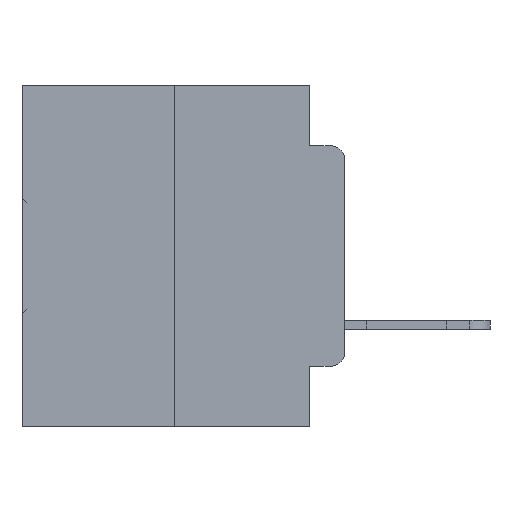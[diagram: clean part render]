
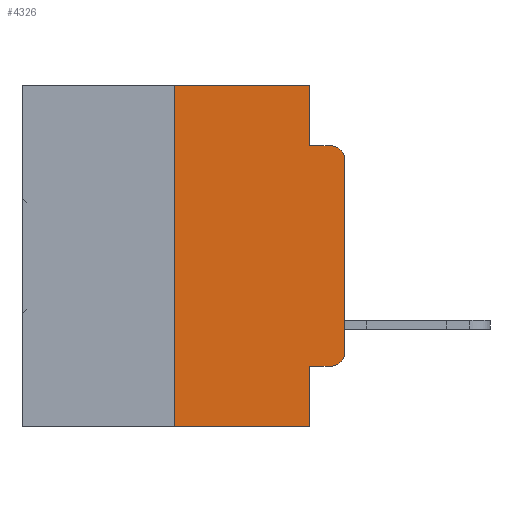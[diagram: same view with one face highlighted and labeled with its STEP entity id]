
A CAD part, left-side view. The second image highlights one B-rep face of the part: STEP entity #4326.
In plain terms, the highlighted planar face has unit normal (-1, 0, 0).
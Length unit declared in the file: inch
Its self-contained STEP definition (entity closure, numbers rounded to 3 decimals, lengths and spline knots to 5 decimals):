
#332 = AXIS2_PLACEMENT_3D ( 'NONE', #28233, #28137, #28130 ) ;
#781 = VECTOR ( 'NONE', #5987, 39.37008 ) ;
#976 = DIRECTION ( 'NONE',  ( 0., -1., 0. ) ) ;
#1057 = CARTESIAN_POINT ( 'NONE',  ( 0., 0.25, -0.5 ) ) ;
#1423 = ORIENTED_EDGE ( 'NONE', *, *, #20901, .F. ) ;
#1630 = CARTESIAN_POINT ( 'NONE',  ( 0., 0., -0.1085 ) ) ;
#2829 = ORIENTED_EDGE ( 'NONE', *, *, #20989, .F. ) ;
#3042 = ORIENTED_EDGE ( 'NONE', *, *, #15015, .F. ) ;
#3251 = EDGE_LOOP ( 'NONE', ( #8736, #9298, #1423, #2829, #3042, #3674, #5039, #5368, #6458, #7933 ) ) ;
#3662 = CARTESIAN_POINT ( 'NONE',  ( 0., 0.051, -0.0885 ) ) ;
#3674 = ORIENTED_EDGE ( 'NONE', *, *, #21372, .F. ) ;
#4326 = ADVANCED_FACE ( 'NONE', ( #28482 ), #28453, .F. ) ;
#5039 = ORIENTED_EDGE ( 'NONE', *, *, #16620, .T. ) ;
#5217 = CARTESIAN_POINT ( 'NONE',  ( 0., 0.473, -0.5 ) ) ;
#5368 = ORIENTED_EDGE ( 'NONE', *, *, #21465, .F. ) ;
#5386 = VECTOR ( 'NONE', #23985, 39.37008 ) ;
#5987 = DIRECTION ( 'NONE',  ( 0., 0., 1. ) ) ;
#6069 = CARTESIAN_POINT ( 'NONE',  ( 0., 0., 0. ) ) ;
#6242 = VECTOR ( 'NONE', #976, 39.37008 ) ;
#6410 = LINE ( 'NONE', #18366, #19585 ) ;
#6458 = ORIENTED_EDGE ( 'NONE', *, *, #21473, .T. ) ;
#7432 = VERTEX_POINT ( 'NONE', #24612 ) ;
#7849 = VERTEX_POINT ( 'NONE', #14392 ) ;
#7933 = ORIENTED_EDGE ( 'NONE', *, *, #21521, .T. ) ;
#8736 = ORIENTED_EDGE ( 'NONE', *, *, #19960, .T. ) ;
#9298 = ORIENTED_EDGE ( 'NONE', *, *, #20774, .T. ) ;
#9593 = VERTEX_POINT ( 'NONE', #23937 ) ;
#9625 = DIRECTION ( 'NONE',  ( -1., 0., 0. ) ) ;
#9706 = CARTESIAN_POINT ( 'NONE',  ( 0., 0.02, -0.1085 ) ) ;
#12135 = CIRCLE ( 'NONE', #24393, 0.02 ) ;
#12314 = VERTEX_POINT ( 'NONE', #20708 ) ;
#12506 = LINE ( 'NONE', #25046, #18585 ) ;
#13305 = VERTEX_POINT ( 'NONE', #1057 ) ;
#13372 = LINE ( 'NONE', #3662, #6242 ) ;
#13394 = CARTESIAN_POINT ( 'NONE',  ( 0., 0.051, -0.4115 ) ) ;
#14392 = CARTESIAN_POINT ( 'NONE',  ( 0., 0.051, 0. ) ) ;
#14623 = DIRECTION ( 'NONE',  ( 0., 0., -1. ) ) ;
#15015 = EDGE_CURVE ( 'NONE', #12314, #7849, #6410, .T. ) ;
#16620 = EDGE_CURVE ( 'NONE', #13305, #19238, #23354, .T. ) ;
#16702 = VECTOR ( 'NONE', #22407, 39.37008 ) ;
#17532 = AXIS2_PLACEMENT_3D ( 'NONE', #22869, #22823, #22817 ) ;
#17819 = CIRCLE ( 'NONE', #17532, 0.02 ) ;
#18154 = DIRECTION ( 'NONE',  ( 0., -1., 0. ) ) ;
#18366 = CARTESIAN_POINT ( 'NONE',  ( 0., 0.473, 0. ) ) ;
#18414 = CARTESIAN_POINT ( 'NONE',  ( 0., 0., -0.3915 ) ) ;
#18585 = VECTOR ( 'NONE', #23670, 39.37008 ) ;
#19238 = VERTEX_POINT ( 'NONE', #19854 ) ;
#19585 = VECTOR ( 'NONE', #18154, 39.37008 ) ;
#19854 = CARTESIAN_POINT ( 'NONE',  ( 0., 0.051, -0.5 ) ) ;
#19960 = EDGE_CURVE ( 'NONE', #23480, #22601, #21810, .T. ) ;
#20708 = CARTESIAN_POINT ( 'NONE',  ( 0., 0.25, 0. ) ) ;
#20774 = EDGE_CURVE ( 'NONE', #22601, #9593, #12135, .T. ) ;
#20901 = EDGE_CURVE ( 'NONE', #7432, #9593, #13372, .T. ) ;
#20960 = VERTEX_POINT ( 'NONE', #32880 ) ;
#20989 = EDGE_CURVE ( 'NONE', #7849, #7432, #30144, .T. ) ;
#21372 = EDGE_CURVE ( 'NONE', #13305, #12314, #28237, .T. ) ;
#21465 = EDGE_CURVE ( 'NONE', #22135, #19238, #25941, .T. ) ;
#21473 = EDGE_CURVE ( 'NONE', #22135, #20960, #12506, .T. ) ;
#21521 = EDGE_CURVE ( 'NONE', #20960, #23480, #17819, .T. ) ;
#21721 = VECTOR ( 'NONE', #25743, 39.37008 ) ;
#21810 = LINE ( 'NONE', #6069, #781 ) ;
#22135 = VERTEX_POINT ( 'NONE', #13394 ) ;
#22407 = DIRECTION ( 'NONE',  ( 0., -1., 0. ) ) ;
#22601 = VERTEX_POINT ( 'NONE', #1630 ) ;
#22817 = DIRECTION ( 'NONE',  ( 0., 0., -1. ) ) ;
#22823 = DIRECTION ( 'NONE',  ( -1., 0., 0. ) ) ;
#22869 = CARTESIAN_POINT ( 'NONE',  ( 0., 0.02, -0.3915 ) ) ;
#23354 = LINE ( 'NONE', #5217, #16702 ) ;
#23480 = VERTEX_POINT ( 'NONE', #18414 ) ;
#23670 = DIRECTION ( 'NONE',  ( 0., -1., 0. ) ) ;
#23680 = VECTOR ( 'NONE', #32076, 39.37008 ) ;
#23937 = CARTESIAN_POINT ( 'NONE',  ( 0., 0.02, -0.0885 ) ) ;
#23985 = DIRECTION ( 'NONE',  ( 0., 0., -1. ) ) ;
#24102 = CARTESIAN_POINT ( 'NONE',  ( 0., 0.051, 0. ) ) ;
#24393 = AXIS2_PLACEMENT_3D ( 'NONE', #9706, #9625, #14623 ) ;
#24612 = CARTESIAN_POINT ( 'NONE',  ( 0., 0.051, -0.0885 ) ) ;
#25046 = CARTESIAN_POINT ( 'NONE',  ( 0., 0.051, -0.4115 ) ) ;
#25681 = CARTESIAN_POINT ( 'NONE',  ( 0., 0.25, 0. ) ) ;
#25743 = DIRECTION ( 'NONE',  ( 0., 0., 1. ) ) ;
#25941 = LINE ( 'NONE', #24102, #5386 ) ;
#28130 = DIRECTION ( 'NONE',  ( 0., 0., -1. ) ) ;
#28137 = DIRECTION ( 'NONE',  ( 1., 0., 0. ) ) ;
#28233 = CARTESIAN_POINT ( 'NONE',  ( 0., 0.473, 0. ) ) ;
#28237 = LINE ( 'NONE', #25681, #21721 ) ;
#28453 = PLANE ( 'NONE',  #332 ) ;
#28482 = FACE_OUTER_BOUND ( 'NONE', #3251, .T. ) ;
#30144 = LINE ( 'NONE', #32212, #23680 ) ;
#32076 = DIRECTION ( 'NONE',  ( 0., 0., -1. ) ) ;
#32212 = CARTESIAN_POINT ( 'NONE',  ( 0., 0.051, 0. ) ) ;
#32880 = CARTESIAN_POINT ( 'NONE',  ( 0., 0.02, -0.4115 ) ) ;
